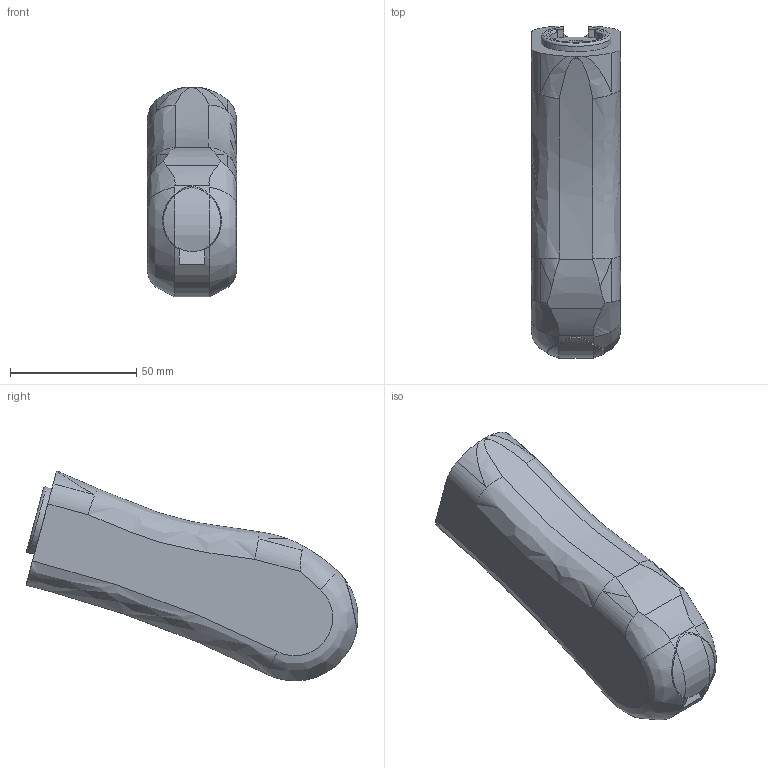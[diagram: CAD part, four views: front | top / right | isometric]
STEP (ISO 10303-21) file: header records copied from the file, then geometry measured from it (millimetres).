
FILE_DESCRIPTION(/* description */ (''),/* implementation_level */ '2;1');
FILE_NAME(/* name */ 'Birdshead Grip.step',/* time_stamp */ '2020-10-31T21:54:54-04:00',/* author */ (''),/* organization */ (''),/* preprocessor_version */ 'ST-DEVELOPER v18.1',/* originating_system */ 'Autodesk Translation Framework v9.3.0.1241',/* authorisation */ '');
FILE_SCHEMA (('AUTOMOTIVE_DESIGN { 1 0 10303 214 3 1 1 }'));
Length unit declared in the file: millimetre
Products named in the file (1): Birdshead Grip
Bounding box: 35.27 x 131.4 x 83.1 mm (x, y, z)
Volume: 182210.4 mm3; surface area: 28250.3 mm2
Topology: 2 solids, 2 shells, 74 faces, 190 edges, 123 vertices
Faces by surface type: plane 30, cylinder 24, bspline 16, torus 3, cone 1
Full cylindrical faces by diameter (mm): 8.5 x1, 13.25 x1, 22.59 x1, 23.25 x1
Entity records: 3517 total; most frequent: CARTESIAN_POINT 1802, ORIENTED_EDGE 380, DIRECTION 304, EDGE_CURVE 190, VERTEX_POINT 123, AXIS2_PLACEMENT_3D 112, LINE 80, VECTOR 80
